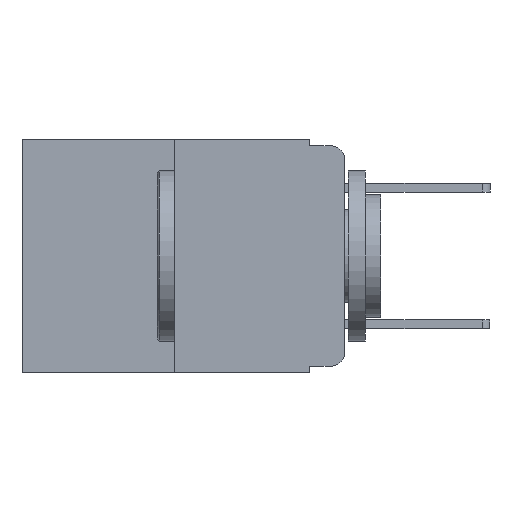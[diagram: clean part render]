
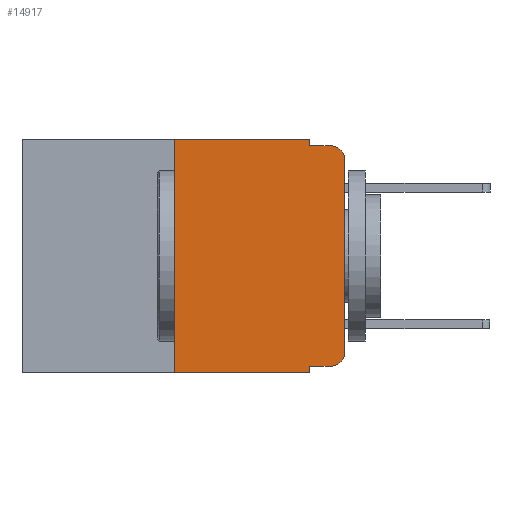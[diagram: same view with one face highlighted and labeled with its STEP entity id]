
A CAD part, left-side view. The second image highlights one B-rep face of the part: STEP entity #14917.
In plain terms, the highlighted planar face has unit normal (-1, 0, 0).
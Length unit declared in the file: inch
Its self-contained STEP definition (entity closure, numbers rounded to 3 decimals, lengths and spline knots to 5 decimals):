
#42 = ORIENTED_EDGE ( 'NONE', *, *, #13177, .F. ) ;
#749 = CARTESIAN_POINT ( 'NONE',  ( 0., 0.051, 0. ) ) ;
#1029 = ORIENTED_EDGE ( 'NONE', *, *, #14817, .F. ) ;
#1310 = ORIENTED_EDGE ( 'NONE', *, *, #3108, .T. ) ;
#1774 = ORIENTED_EDGE ( 'NONE', *, *, #7359, .T. ) ;
#1779 = VERTEX_POINT ( 'NONE', #13813 ) ;
#1827 = ORIENTED_EDGE ( 'NONE', *, *, #6392, .F. ) ;
#2116 = ORIENTED_EDGE ( 'NONE', *, *, #17533, .F. ) ;
#2117 = VERTEX_POINT ( 'NONE', #14515 ) ;
#2232 = VERTEX_POINT ( 'NONE', #23180 ) ;
#2458 = LINE ( 'NONE', #20858, #21645 ) ;
#2531 = CARTESIAN_POINT ( 'NONE',  ( 0., 0.02, -0.03 ) ) ;
#2787 = ORIENTED_EDGE ( 'NONE', *, *, #7406, .T. ) ;
#3108 = EDGE_CURVE ( 'NONE', #5556, #21715, #22783, .T. ) ;
#3245 = ORIENTED_EDGE ( 'NONE', *, *, #10425, .F. ) ;
#3614 = ORIENTED_EDGE ( 'NONE', *, *, #22039, .T. ) ;
#3650 = AXIS2_PLACEMENT_3D ( 'NONE', #7243, #20367, #9187 ) ;
#3860 = CIRCLE ( 'NONE', #21414, 0.02 ) ;
#3997 = ORIENTED_EDGE ( 'NONE', *, *, #12869, .T. ) ;
#4075 = CARTESIAN_POINT ( 'NONE',  ( 0., 0.473, 0. ) ) ;
#4131 = LINE ( 'NONE', #23460, #19930 ) ;
#4248 = CARTESIAN_POINT ( 'NONE',  ( 0., 0.051, -0.01 ) ) ;
#4566 = VECTOR ( 'NONE', #9007, 39.37008 ) ;
#4648 = DIRECTION ( 'NONE',  ( 0., 0., -1. ) ) ;
#4741 = DIRECTION ( 'NONE',  ( 0., -1., 0. ) ) ;
#5143 = VECTOR ( 'NONE', #11371, 39.37008 ) ;
#5556 = VERTEX_POINT ( 'NONE', #8343 ) ;
#5567 = CIRCLE ( 'NONE', #3650, 0.02 ) ;
#6140 = DIRECTION ( 'NONE',  ( 0., 0., -1. ) ) ;
#6313 = DIRECTION ( 'NONE',  ( 0., -1., 0. ) ) ;
#6392 = EDGE_CURVE ( 'NONE', #13904, #12399, #14667, .T. ) ;
#6685 = CARTESIAN_POINT ( 'NONE',  ( 0., 0.473, -0.343 ) ) ;
#7243 = CARTESIAN_POINT ( 'NONE',  ( 0., 0.02, -0.313 ) ) ;
#7359 = EDGE_CURVE ( 'NONE', #2232, #1779, #3860, .T. ) ;
#7406 = EDGE_CURVE ( 'NONE', #16918, #20640, #8557, .T. ) ;
#7462 = VECTOR ( 'NONE', #6313, 39.37008 ) ;
#8343 = CARTESIAN_POINT ( 'NONE',  ( 0., 0.051, -0.333 ) ) ;
#8557 = LINE ( 'NONE', #6685, #18491 ) ;
#8976 = CARTESIAN_POINT ( 'NONE',  ( 0., 0.051, 0. ) ) ;
#9007 = DIRECTION ( 'NONE',  ( 0., 0., -1. ) ) ;
#9115 = CARTESIAN_POINT ( 'NONE',  ( 0., 0.051, -0.343 ) ) ;
#9187 = DIRECTION ( 'NONE',  ( 0., 0., -1. ) ) ;
#10425 = EDGE_CURVE ( 'NONE', #12399, #1779, #11847, .T. ) ;
#11371 = DIRECTION ( 'NONE',  ( 0., 0., 1. ) ) ;
#11594 = DIRECTION ( 'NONE',  ( 0., -1., 0. ) ) ;
#11774 = PLANE ( 'NONE',  #23136 ) ;
#11847 = LINE ( 'NONE', #4248, #7462 ) ;
#12006 = CARTESIAN_POINT ( 'NONE',  ( 0., 0.25, -0.343 ) ) ;
#12399 = VERTEX_POINT ( 'NONE', #24548 ) ;
#12869 = EDGE_CURVE ( 'NONE', #2117, #2232, #20230, .T. ) ;
#13177 = EDGE_CURVE ( 'NONE', #16918, #22303, #4131, .T. ) ;
#13535 = CARTESIAN_POINT ( 'NONE',  ( 0., 0.051, -0.333 ) ) ;
#13813 = CARTESIAN_POINT ( 'NONE',  ( 0., 0.02, -0.01 ) ) ;
#13904 = VERTEX_POINT ( 'NONE', #749 ) ;
#14515 = CARTESIAN_POINT ( 'NONE',  ( 0., 0., -0.313 ) ) ;
#14667 = LINE ( 'NONE', #8976, #4566 ) ;
#14817 = EDGE_CURVE ( 'NONE', #22303, #13904, #2458, .T. ) ;
#14917 = ADVANCED_FACE ( 'NONE', ( #24266 ), #11774, .F. ) ;
#15619 = CARTESIAN_POINT ( 'NONE',  ( 0., 0.051, 0. ) ) ;
#16005 = DIRECTION ( 'NONE',  ( -1., 0., 0. ) ) ;
#16436 = EDGE_LOOP ( 'NONE', ( #3997, #1774, #3245, #1827, #1029, #42, #2787, #2116, #1310, #3614 ) ) ;
#16918 = VERTEX_POINT ( 'NONE', #12006 ) ;
#17402 = DIRECTION ( 'NONE',  ( 1., 0., 0. ) ) ;
#17533 = EDGE_CURVE ( 'NONE', #5556, #20640, #23878, .T. ) ;
#17790 = VECTOR ( 'NONE', #19349, 39.37008 ) ;
#17882 = DIRECTION ( 'NONE',  ( 0., 0., 1. ) ) ;
#18491 = VECTOR ( 'NONE', #4741, 39.37008 ) ;
#18732 = CARTESIAN_POINT ( 'NONE',  ( 0., 0.25, 0. ) ) ;
#18902 = VECTOR ( 'NONE', #23199, 39.37008 ) ;
#19349 = DIRECTION ( 'NONE',  ( 0., -1., 0. ) ) ;
#19930 = VECTOR ( 'NONE', #17882, 39.37008 ) ;
#20230 = LINE ( 'NONE', #22657, #5143 ) ;
#20367 = DIRECTION ( 'NONE',  ( -1., 0., 0. ) ) ;
#20640 = VERTEX_POINT ( 'NONE', #9115 ) ;
#20858 = CARTESIAN_POINT ( 'NONE',  ( 0., 0.473, 0. ) ) ;
#21199 = CARTESIAN_POINT ( 'NONE',  ( 0., 0.02, -0.333 ) ) ;
#21414 = AXIS2_PLACEMENT_3D ( 'NONE', #2531, #16005, #4648 ) ;
#21645 = VECTOR ( 'NONE', #11594, 39.37008 ) ;
#21715 = VERTEX_POINT ( 'NONE', #21199 ) ;
#22039 = EDGE_CURVE ( 'NONE', #21715, #2117, #5567, .T. ) ;
#22303 = VERTEX_POINT ( 'NONE', #18732 ) ;
#22657 = CARTESIAN_POINT ( 'NONE',  ( 0., 0., 0. ) ) ;
#22783 = LINE ( 'NONE', #13535, #17790 ) ;
#23136 = AXIS2_PLACEMENT_3D ( 'NONE', #4075, #17402, #6140 ) ;
#23180 = CARTESIAN_POINT ( 'NONE',  ( 0., 0., -0.03 ) ) ;
#23199 = DIRECTION ( 'NONE',  ( 0., 0., -1. ) ) ;
#23460 = CARTESIAN_POINT ( 'NONE',  ( 0., 0.25, 0. ) ) ;
#23878 = LINE ( 'NONE', #15619, #18902 ) ;
#24266 = FACE_OUTER_BOUND ( 'NONE', #16436, .T. ) ;
#24548 = CARTESIAN_POINT ( 'NONE',  ( 0., 0.051, -0.01 ) ) ;
